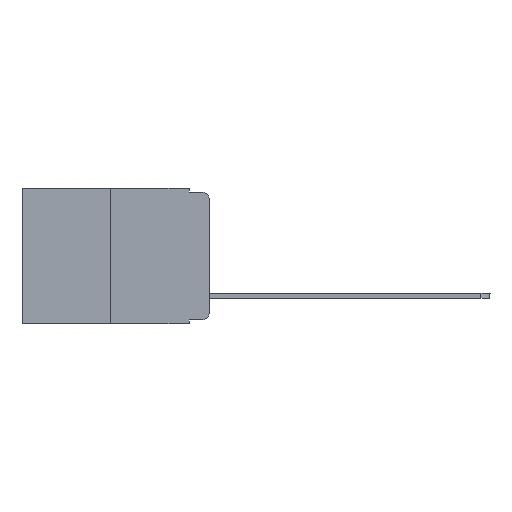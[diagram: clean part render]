
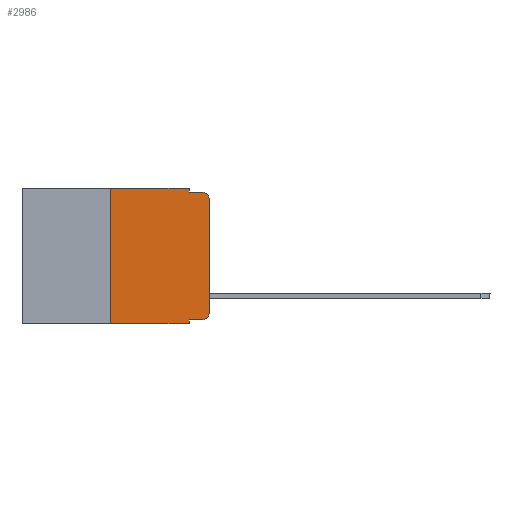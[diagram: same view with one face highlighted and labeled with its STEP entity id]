
A CAD part, left-side view. The second image highlights one B-rep face of the part: STEP entity #2986.
In plain terms, the highlighted planar face has unit normal (-1, 0, 0).
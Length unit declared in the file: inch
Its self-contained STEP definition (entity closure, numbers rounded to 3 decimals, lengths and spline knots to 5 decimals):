
#4 = LINE ( 'NONE', #1798, #5347 ) ;
#16 = VECTOR ( 'NONE', #2394, 39.37008 ) ;
#58 = LINE ( 'NONE', #5054, #7131 ) ;
#93 = LINE ( 'NONE', #3405, #8682 ) ;
#371 = VECTOR ( 'NONE', #6844, 39.37008 ) ;
#644 = EDGE_CURVE ( 'NONE', #2231, #7326, #6518, .T. ) ;
#824 = CARTESIAN_POINT ( 'NONE',  ( 0., 0.02, -0.01 ) ) ;
#867 = CARTESIAN_POINT ( 'NONE',  ( 0., 0.051, -0.333 ) ) ;
#886 = EDGE_LOOP ( 'NONE', ( #6058, #936, #6233, #6072, #8864, #5375, #2124, #1269, #9541, #2955 ) ) ;
#936 = ORIENTED_EDGE ( 'NONE', *, *, #644, .T. ) ;
#1010 = LINE ( 'NONE', #6616, #2109 ) ;
#1108 = VERTEX_POINT ( 'NONE', #867 ) ;
#1269 = ORIENTED_EDGE ( 'NONE', *, *, #7813, .F. ) ;
#1653 = EDGE_CURVE ( 'NONE', #9670, #2231, #8121, .T. ) ;
#1706 = VECTOR ( 'NONE', #6610, 39.37008 ) ;
#1798 = CARTESIAN_POINT ( 'NONE',  ( 0., 0.473, 0. ) ) ;
#2096 = CARTESIAN_POINT ( 'NONE',  ( 0., 0.02, -0.333 ) ) ;
#2109 = VECTOR ( 'NONE', #9925, 39.37008 ) ;
#2117 = AXIS2_PLACEMENT_3D ( 'NONE', #10085, #3423, #8411 ) ;
#2124 = ORIENTED_EDGE ( 'NONE', *, *, #9031, .T. ) ;
#2231 = VERTEX_POINT ( 'NONE', #10124 ) ;
#2394 = DIRECTION ( 'NONE',  ( 0., -1., 0. ) ) ;
#2418 = CARTESIAN_POINT ( 'NONE',  ( 0., 0., -0.313 ) ) ;
#2561 = CARTESIAN_POINT ( 'NONE',  ( 0., 0.25, -0.343 ) ) ;
#2657 = FACE_OUTER_BOUND ( 'NONE', #886, .T. ) ;
#2765 = VECTOR ( 'NONE', #5863, 39.37008 ) ;
#2917 = EDGE_CURVE ( 'NONE', #4932, #8300, #58, .T. ) ;
#2955 = ORIENTED_EDGE ( 'NONE', *, *, #5152, .T. ) ;
#2977 = CIRCLE ( 'NONE', #10576, 0.02 ) ;
#2986 = ADVANCED_FACE ( 'NONE', ( #2657 ), #5911, .F. ) ;
#3078 = LINE ( 'NONE', #5519, #371 ) ;
#3373 = DIRECTION ( 'NONE',  ( 0., 0., -1. ) ) ;
#3405 = CARTESIAN_POINT ( 'NONE',  ( 0., 0.051, -0.333 ) ) ;
#3423 = DIRECTION ( 'NONE',  ( 1., 0., 0. ) ) ;
#3488 = LINE ( 'NONE', #10674, #2765 ) ;
#3929 = AXIS2_PLACEMENT_3D ( 'NONE', #7511, #10001, #4104 ) ;
#4104 = DIRECTION ( 'NONE',  ( 0., 0., -1. ) ) ;
#4152 = LINE ( 'NONE', #9778, #16 ) ;
#4348 = VERTEX_POINT ( 'NONE', #8313 ) ;
#4753 = EDGE_CURVE ( 'NONE', #9134, #8231, #1010, .T. ) ;
#4891 = EDGE_CURVE ( 'NONE', #8300, #7326, #3078, .T. ) ;
#4932 = VERTEX_POINT ( 'NONE', #10596 ) ;
#5054 = CARTESIAN_POINT ( 'NONE',  ( 0., 0.051, 0. ) ) ;
#5152 = EDGE_CURVE ( 'NONE', #7722, #9670, #2977, .T. ) ;
#5347 = VECTOR ( 'NONE', #8420, 39.37008 ) ;
#5375 = ORIENTED_EDGE ( 'NONE', *, *, #4753, .F. ) ;
#5519 = CARTESIAN_POINT ( 'NONE',  ( 0., 0.051, -0.01 ) ) ;
#5689 = CARTESIAN_POINT ( 'NONE',  ( 0., 0., 0. ) ) ;
#5863 = DIRECTION ( 'NONE',  ( 0., 0., -1. ) ) ;
#5911 = PLANE ( 'NONE',  #2117 ) ;
#6058 = ORIENTED_EDGE ( 'NONE', *, *, #1653, .T. ) ;
#6072 = ORIENTED_EDGE ( 'NONE', *, *, #2917, .F. ) ;
#6233 = ORIENTED_EDGE ( 'NONE', *, *, #4891, .F. ) ;
#6518 = CIRCLE ( 'NONE', #3929, 0.02 ) ;
#6610 = DIRECTION ( 'NONE',  ( 0., 0., 1. ) ) ;
#6616 = CARTESIAN_POINT ( 'NONE',  ( 0., 0.25, 0. ) ) ;
#6723 = CARTESIAN_POINT ( 'NONE',  ( 0., 0.25, 0. ) ) ;
#6844 = DIRECTION ( 'NONE',  ( 0., -1., 0. ) ) ;
#6871 = DIRECTION ( 'NONE',  ( -1., 0., 0. ) ) ;
#6891 = CARTESIAN_POINT ( 'NONE',  ( 0., 0.051, -0.01 ) ) ;
#7131 = VECTOR ( 'NONE', #3373, 39.37008 ) ;
#7326 = VERTEX_POINT ( 'NONE', #824 ) ;
#7511 = CARTESIAN_POINT ( 'NONE',  ( 0., 0.02, -0.03 ) ) ;
#7681 = CARTESIAN_POINT ( 'NONE',  ( 0., 0.02, -0.313 ) ) ;
#7722 = VERTEX_POINT ( 'NONE', #2096 ) ;
#7813 = EDGE_CURVE ( 'NONE', #1108, #4348, #3488, .T. ) ;
#8121 = LINE ( 'NONE', #5689, #1706 ) ;
#8231 = VERTEX_POINT ( 'NONE', #6723 ) ;
#8300 = VERTEX_POINT ( 'NONE', #6891 ) ;
#8313 = CARTESIAN_POINT ( 'NONE',  ( 0., 0.051, -0.343 ) ) ;
#8411 = DIRECTION ( 'NONE',  ( 0., 0., -1. ) ) ;
#8420 = DIRECTION ( 'NONE',  ( 0., -1., 0. ) ) ;
#8647 = EDGE_CURVE ( 'NONE', #1108, #7722, #93, .T. ) ;
#8682 = VECTOR ( 'NONE', #9199, 39.37008 ) ;
#8864 = ORIENTED_EDGE ( 'NONE', *, *, #10288, .F. ) ;
#9031 = EDGE_CURVE ( 'NONE', #9134, #4348, #4152, .T. ) ;
#9134 = VERTEX_POINT ( 'NONE', #2561 ) ;
#9199 = DIRECTION ( 'NONE',  ( 0., -1., 0. ) ) ;
#9541 = ORIENTED_EDGE ( 'NONE', *, *, #8647, .T. ) ;
#9670 = VERTEX_POINT ( 'NONE', #2418 ) ;
#9778 = CARTESIAN_POINT ( 'NONE',  ( 0., 0.473, -0.343 ) ) ;
#9925 = DIRECTION ( 'NONE',  ( 0., 0., 1. ) ) ;
#10001 = DIRECTION ( 'NONE',  ( -1., 0., 0. ) ) ;
#10085 = CARTESIAN_POINT ( 'NONE',  ( 0., 0.473, 0. ) ) ;
#10124 = CARTESIAN_POINT ( 'NONE',  ( 0., 0., -0.03 ) ) ;
#10217 = DIRECTION ( 'NONE',  ( 0., 0., -1. ) ) ;
#10288 = EDGE_CURVE ( 'NONE', #8231, #4932, #4, .T. ) ;
#10576 = AXIS2_PLACEMENT_3D ( 'NONE', #7681, #6871, #10217 ) ;
#10596 = CARTESIAN_POINT ( 'NONE',  ( 0., 0.051, 0. ) ) ;
#10674 = CARTESIAN_POINT ( 'NONE',  ( 0., 0.051, 0. ) ) ;
